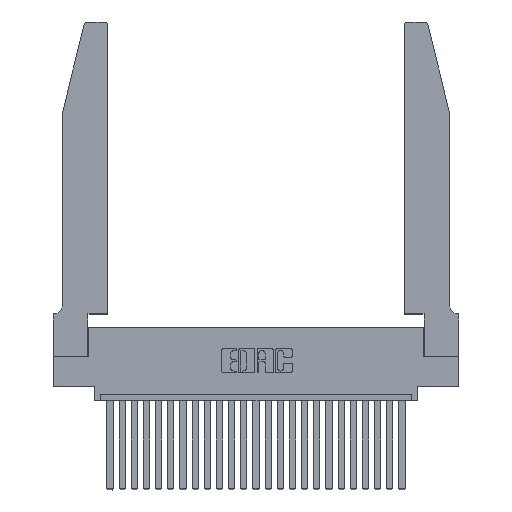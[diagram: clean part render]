
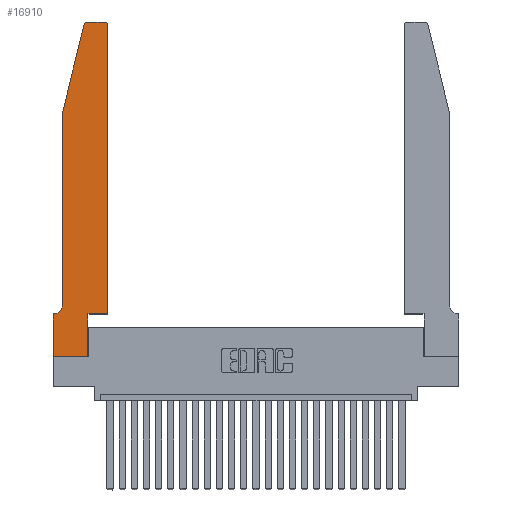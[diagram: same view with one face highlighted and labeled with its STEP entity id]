
A CAD part, top view. The second image highlights one B-rep face of the part: STEP entity #16910.
In plain terms, the highlighted planar face has unit normal (0, 0, 1).
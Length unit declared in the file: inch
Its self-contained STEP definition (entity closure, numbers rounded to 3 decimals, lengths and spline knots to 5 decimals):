
#283 = DIRECTION ( 'NONE',  ( 0., -1., 0. ) ) ;
#438 = CARTESIAN_POINT ( 'NONE',  ( 0.2865, 0., 0.37 ) ) ;
#551 = EDGE_CURVE ( 'NONE', #1730, #20084, #15306, .T. ) ;
#588 = EDGE_CURVE ( 'NONE', #9069, #25752, #13732, .T. ) ;
#629 = DIRECTION ( 'NONE',  ( -0.239, -0.971, 0. ) ) ;
#801 = VERTEX_POINT ( 'NONE', #16439 ) ;
#914 = PLANE ( 'NONE',  #1189 ) ;
#1189 = AXIS2_PLACEMENT_3D ( 'NONE', #2919, #16795, #16552 ) ;
#1708 = CARTESIAN_POINT ( 'NONE',  ( 0.4205, 2.75, 0.37 ) ) ;
#1730 = VERTEX_POINT ( 'NONE', #18618 ) ;
#1876 = EDGE_CURVE ( 'NONE', #20084, #4181, #2670, .T. ) ;
#2076 = VERTEX_POINT ( 'NONE', #4540 ) ;
#2205 = ORIENTED_EDGE ( 'NONE', *, *, #14040, .T. ) ;
#2206 = CARTESIAN_POINT ( 'NONE',  ( 0.0055, 0.35, 0.37 ) ) ;
#2418 = LINE ( 'NONE', #3344, #12119 ) ;
#2662 = CARTESIAN_POINT ( 'NONE',  ( 0.4505, 2.72, 0.37 ) ) ;
#2670 = CIRCLE ( 'NONE', #13534, 0.07 ) ;
#2919 = CARTESIAN_POINT ( 'NONE',  ( 0., 0.35, 0.37 ) ) ;
#3344 = CARTESIAN_POINT ( 'NONE',  ( 0., 0., 0.37 ) ) ;
#4181 = VERTEX_POINT ( 'NONE', #2206 ) ;
#4387 = VECTOR ( 'NONE', #21536, 39.37008 ) ;
#4540 = CARTESIAN_POINT ( 'NONE',  ( 0., 0.35, 0.37 ) ) ;
#5091 = AXIS2_PLACEMENT_3D ( 'NONE', #13084, #10848, #7119 ) ;
#5167 = CARTESIAN_POINT ( 'NONE',  ( 0., 0., 0.37 ) ) ;
#5302 = CIRCLE ( 'NONE', #13275, 0.03 ) ;
#5320 = VECTOR ( 'NONE', #283, 39.37008 ) ;
#5393 = ORIENTED_EDGE ( 'NONE', *, *, #23241, .T. ) ;
#5394 = DIRECTION ( 'NONE',  ( 0., 0., 1. ) ) ;
#5551 = VECTOR ( 'NONE', #629, 39.37008 ) ;
#5966 = ORIENTED_EDGE ( 'NONE', *, *, #1876, .T. ) ;
#6067 = CARTESIAN_POINT ( 'NONE',  ( 0.2865, 0.35, 0.37 ) ) ;
#6213 = CARTESIAN_POINT ( 'NONE',  ( 0.0055, 0.42, 0.37 ) ) ;
#6407 = EDGE_CURVE ( 'NONE', #16647, #9069, #2418, .T. ) ;
#7119 = DIRECTION ( 'NONE',  ( 1., 0., 0. ) ) ;
#8291 = LINE ( 'NONE', #5167, #10795 ) ;
#8450 = VECTOR ( 'NONE', #12157, 39.37008 ) ;
#8907 = EDGE_CURVE ( 'NONE', #2076, #16647, #8291, .T. ) ;
#9069 = VERTEX_POINT ( 'NONE', #438 ) ;
#9367 = LINE ( 'NONE', #12490, #19636 ) ;
#9438 = DIRECTION ( 'NONE',  ( 1., 0., 0. ) ) ;
#9628 = CARTESIAN_POINT ( 'NONE',  ( 0.0755, 0.35, 0.37 ) ) ;
#10305 = DIRECTION ( 'NONE',  ( 0., 0., -1. ) ) ;
#10307 = EDGE_CURVE ( 'NONE', #16208, #13455, #10731, .T. ) ;
#10643 = CARTESIAN_POINT ( 'NONE',  ( 0.2865, 0.35, 0.37 ) ) ;
#10729 = ORIENTED_EDGE ( 'NONE', *, *, #6407, .T. ) ;
#10731 = LINE ( 'NONE', #18386, #24704 ) ;
#10795 = VECTOR ( 'NONE', #15452, 39.37008 ) ;
#10848 = DIRECTION ( 'NONE',  ( 0., 0., 1. ) ) ;
#10980 = DIRECTION ( 'NONE',  ( 1., 0., 0. ) ) ;
#12119 = VECTOR ( 'NONE', #9438, 39.37008 ) ;
#12157 = DIRECTION ( 'NONE',  ( 0., 1., 0. ) ) ;
#12337 = EDGE_CURVE ( 'NONE', #25752, #22009, #21510, .T. ) ;
#12490 = CARTESIAN_POINT ( 'NONE',  ( 0.4505, 0.35, 0.37 ) ) ;
#13084 = CARTESIAN_POINT ( 'NONE',  ( 0.284, 2.72, 0.37 ) ) ;
#13275 = AXIS2_PLACEMENT_3D ( 'NONE', #21066, #5394, #10980 ) ;
#13455 = VERTEX_POINT ( 'NONE', #13527 ) ;
#13527 = CARTESIAN_POINT ( 'NONE',  ( 0.284, 2.75, 0.37 ) ) ;
#13534 = AXIS2_PLACEMENT_3D ( 'NONE', #6213, #10305, #14760 ) ;
#13732 = LINE ( 'NONE', #6067, #8450 ) ;
#13808 = DIRECTION ( 'NONE',  ( -1., 0., 0. ) ) ;
#14040 = EDGE_CURVE ( 'NONE', #4181, #2076, #25436, .T. ) ;
#14760 = DIRECTION ( 'NONE',  ( -1., 0., 0. ) ) ;
#15071 = ORIENTED_EDGE ( 'NONE', *, *, #10307, .T. ) ;
#15306 = LINE ( 'NONE', #19476, #5320 ) ;
#15452 = DIRECTION ( 'NONE',  ( 0., -1., 0. ) ) ;
#15461 = CARTESIAN_POINT ( 'NONE',  ( 0.4505, 0.35, 0.37 ) ) ;
#15661 = ORIENTED_EDGE ( 'NONE', *, *, #551, .T. ) ;
#16208 = VERTEX_POINT ( 'NONE', #1708 ) ;
#16384 = ORIENTED_EDGE ( 'NONE', *, *, #588, .T. ) ;
#16439 = CARTESIAN_POINT ( 'NONE',  ( 0.25487, 2.72718, 0.37 ) ) ;
#16442 = ORIENTED_EDGE ( 'NONE', *, *, #21921, .T. ) ;
#16521 = CARTESIAN_POINT ( 'NONE',  ( 0.0755, 2., 0.37 ) ) ;
#16552 = DIRECTION ( 'NONE',  ( 1., 0., 0. ) ) ;
#16576 = DIRECTION ( 'NONE',  ( -1., 0., 0. ) ) ;
#16647 = VERTEX_POINT ( 'NONE', #19750 ) ;
#16795 = DIRECTION ( 'NONE',  ( 0., 0., 1. ) ) ;
#16810 = CIRCLE ( 'NONE', #5091, 0.03 ) ;
#16910 = ADVANCED_FACE ( 'NONE', ( #24112 ), #914, .T. ) ;
#18386 = CARTESIAN_POINT ( 'NONE',  ( 0.2605, 2.75, 0.37 ) ) ;
#18404 = EDGE_LOOP ( 'NONE', ( #15071, #24691, #5393, #15661, #5966, #2205, #19965, #10729, #16384, #18716, #16442, #19231 ) ) ;
#18550 = CARTESIAN_POINT ( 'NONE',  ( 0.4505, 0.35, 0.37 ) ) ;
#18618 = CARTESIAN_POINT ( 'NONE',  ( 0.0755, 2., 0.37 ) ) ;
#18716 = ORIENTED_EDGE ( 'NONE', *, *, #12337, .T. ) ;
#19231 = ORIENTED_EDGE ( 'NONE', *, *, #22147, .T. ) ;
#19476 = CARTESIAN_POINT ( 'NONE',  ( 0.0755, 2., 0.37 ) ) ;
#19636 = VECTOR ( 'NONE', #25339, 39.37008 ) ;
#19750 = CARTESIAN_POINT ( 'NONE',  ( 0., 0., 0.37 ) ) ;
#19965 = ORIENTED_EDGE ( 'NONE', *, *, #8907, .T. ) ;
#20084 = VERTEX_POINT ( 'NONE', #23993 ) ;
#20201 = LINE ( 'NONE', #16521, #5551 ) ;
#20370 = EDGE_CURVE ( 'NONE', #13455, #801, #16810, .T. ) ;
#21066 = CARTESIAN_POINT ( 'NONE',  ( 0.4205, 2.72, 0.37 ) ) ;
#21510 = LINE ( 'NONE', #15461, #4387 ) ;
#21536 = DIRECTION ( 'NONE',  ( 1., 0., 0. ) ) ;
#21921 = EDGE_CURVE ( 'NONE', #22009, #22596, #9367, .T. ) ;
#22009 = VERTEX_POINT ( 'NONE', #18550 ) ;
#22147 = EDGE_CURVE ( 'NONE', #22596, #16208, #5302, .T. ) ;
#22596 = VERTEX_POINT ( 'NONE', #2662 ) ;
#23241 = EDGE_CURVE ( 'NONE', #801, #1730, #20201, .T. ) ;
#23993 = CARTESIAN_POINT ( 'NONE',  ( 0.0755, 0.42, 0.37 ) ) ;
#24112 = FACE_OUTER_BOUND ( 'NONE', #18404, .T. ) ;
#24691 = ORIENTED_EDGE ( 'NONE', *, *, #20370, .T. ) ;
#24704 = VECTOR ( 'NONE', #16576, 39.37008 ) ;
#25339 = DIRECTION ( 'NONE',  ( 0., 1., 0. ) ) ;
#25436 = LINE ( 'NONE', #9628, #25751 ) ;
#25751 = VECTOR ( 'NONE', #13808, 39.37008 ) ;
#25752 = VERTEX_POINT ( 'NONE', #10643 ) ;
